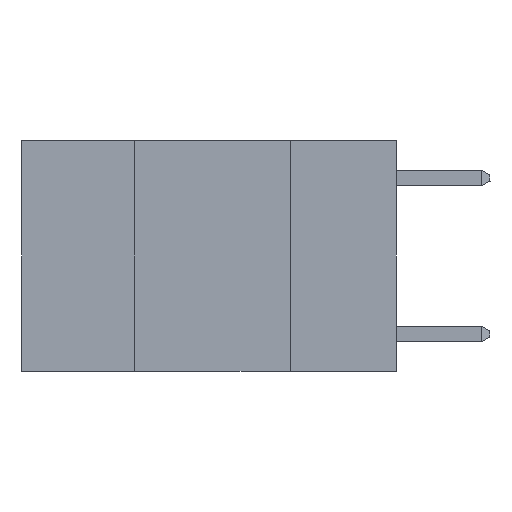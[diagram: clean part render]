
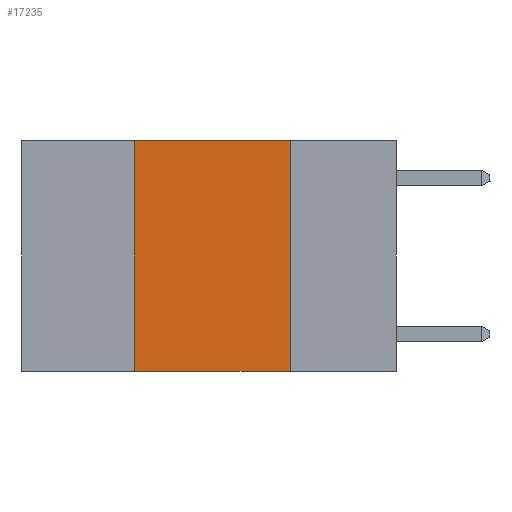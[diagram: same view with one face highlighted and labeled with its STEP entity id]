
A CAD part, left-side view. The second image highlights one B-rep face of the part: STEP entity #17235.
In plain terms, the highlighted planar face has unit normal (-1, 0, 0).
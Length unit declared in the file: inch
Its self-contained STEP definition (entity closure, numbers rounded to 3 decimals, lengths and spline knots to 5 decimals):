
#621 = DIRECTION ( 'NONE',  ( 0., 0., -1. ) ) ;
#881 = LINE ( 'NONE', #16866, #9560 ) ;
#2416 = FACE_OUTER_BOUND ( 'NONE', #19841, .T. ) ;
#2613 = DIRECTION ( 'NONE',  ( 0., -1., 0. ) ) ;
#2828 = LINE ( 'NONE', #7009, #18690 ) ;
#4400 = ORIENTED_EDGE ( 'NONE', *, *, #18868, .F. ) ;
#4973 = ORIENTED_EDGE ( 'NONE', *, *, #9201, .F. ) ;
#5253 = EDGE_CURVE ( 'NONE', #12915, #6077, #2828, .T. ) ;
#5511 = PLANE ( 'NONE',  #16291 ) ;
#6023 = VERTEX_POINT ( 'NONE', #6981 ) ;
#6077 = VERTEX_POINT ( 'NONE', #15088 ) ;
#6981 = CARTESIAN_POINT ( 'NONE',  ( 0., 0.17, -0.37 ) ) ;
#7009 = CARTESIAN_POINT ( 'NONE',  ( 0., 0.42, 0. ) ) ;
#7170 = CARTESIAN_POINT ( 'NONE',  ( 0., 0.6, 0. ) ) ;
#7544 = ORIENTED_EDGE ( 'NONE', *, *, #5253, .F. ) ;
#7793 = ORIENTED_EDGE ( 'NONE', *, *, #13153, .T. ) ;
#8603 = CARTESIAN_POINT ( 'NONE',  ( 0., 0.42, -0.37 ) ) ;
#8754 = DIRECTION ( 'NONE',  ( 0., -1., 0. ) ) ;
#9201 = EDGE_CURVE ( 'NONE', #19952, #6023, #881, .T. ) ;
#9560 = VECTOR ( 'NONE', #10660, 39.37008 ) ;
#10379 = DIRECTION ( 'NONE',  ( 1., 0., 0. ) ) ;
#10660 = DIRECTION ( 'NONE',  ( 0., 0., -1. ) ) ;
#10743 = VECTOR ( 'NONE', #8754, 39.37008 ) ;
#11255 = LINE ( 'NONE', #7170, #10743 ) ;
#11383 = VECTOR ( 'NONE', #2613, 39.37008 ) ;
#11872 = LINE ( 'NONE', #12313, #11383 ) ;
#12313 = CARTESIAN_POINT ( 'NONE',  ( 0., 0.6, -0.37 ) ) ;
#12915 = VERTEX_POINT ( 'NONE', #8603 ) ;
#13153 = EDGE_CURVE ( 'NONE', #12915, #6023, #11872, .T. ) ;
#13329 = CARTESIAN_POINT ( 'NONE',  ( 0., 0.17, 0. ) ) ;
#15088 = CARTESIAN_POINT ( 'NONE',  ( 0., 0.42, 0. ) ) ;
#16291 = AXIS2_PLACEMENT_3D ( 'NONE', #19614, #10379, #621 ) ;
#16866 = CARTESIAN_POINT ( 'NONE',  ( 0., 0.17, 0. ) ) ;
#17235 = ADVANCED_FACE ( 'NONE', ( #2416 ), #5511, .F. ) ;
#18690 = VECTOR ( 'NONE', #19491, 39.37008 ) ;
#18868 = EDGE_CURVE ( 'NONE', #6077, #19952, #11255, .T. ) ;
#19491 = DIRECTION ( 'NONE',  ( 0., 0., 1. ) ) ;
#19614 = CARTESIAN_POINT ( 'NONE',  ( 0., 0.6, 0. ) ) ;
#19841 = EDGE_LOOP ( 'NONE', ( #4973, #4400, #7544, #7793 ) ) ;
#19952 = VERTEX_POINT ( 'NONE', #13329 ) ;
